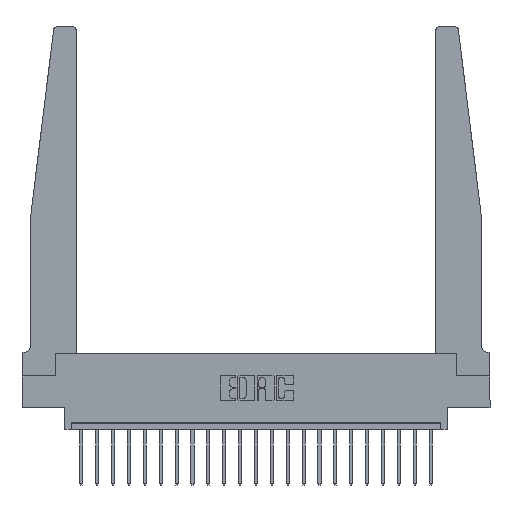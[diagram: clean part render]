
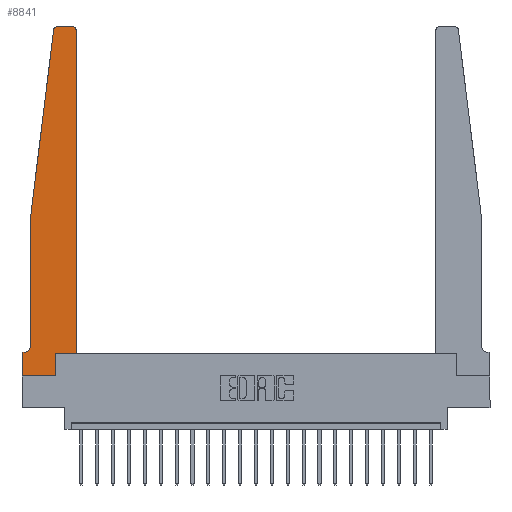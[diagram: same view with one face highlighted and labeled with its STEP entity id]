
A CAD part, top view. The second image highlights one B-rep face of the part: STEP entity #8841.
In plain terms, the highlighted planar face has unit normal (0, 0, 1).
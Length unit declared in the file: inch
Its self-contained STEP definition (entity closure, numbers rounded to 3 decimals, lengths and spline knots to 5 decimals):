
#238 = VECTOR ( 'NONE', #19672, 39.37008 ) ;
#254 = CARTESIAN_POINT ( 'NONE',  ( 0.065, 0.1875, 0.37 ) ) ;
#684 = CARTESIAN_POINT ( 'NONE',  ( 0.425, 0.18, 0.37 ) ) ;
#1809 = LINE ( 'NONE', #3387, #8840 ) ;
#2019 = LINE ( 'NONE', #8628, #5111 ) ;
#2046 = DIRECTION ( 'NONE',  ( 0., 1., 0. ) ) ;
#2198 = EDGE_CURVE ( 'NONE', #18821, #7153, #13182, .T. ) ;
#2210 = CARTESIAN_POINT ( 'NONE',  ( 0., 0.1875, 0.37 ) ) ;
#2639 = CARTESIAN_POINT ( 'NONE',  ( 0.065, 1.25, 0.37 ) ) ;
#3086 = CARTESIAN_POINT ( 'NONE',  ( 0., 0., 0.37 ) ) ;
#3207 = EDGE_CURVE ( 'NONE', #20640, #17232, #13992, .T. ) ;
#3245 = EDGE_CURVE ( 'NONE', #11460, #18821, #2019, .T. ) ;
#3387 = CARTESIAN_POINT ( 'NONE',  ( 0., 0., 0.37 ) ) ;
#3654 = CARTESIAN_POINT ( 'NONE',  ( 0.425, 0.18, 0.37 ) ) ;
#3696 = ORIENTED_EDGE ( 'NONE', *, *, #17014, .T. ) ;
#4176 = VERTEX_POINT ( 'NONE', #3654 ) ;
#4183 = ORIENTED_EDGE ( 'NONE', *, *, #4213, .T. ) ;
#4193 = CARTESIAN_POINT ( 'NONE',  ( 0., 0., 0.37 ) ) ;
#4213 = EDGE_CURVE ( 'NONE', #21275, #11460, #18660, .T. ) ;
#4415 = VECTOR ( 'NONE', #19934, 39.37008 ) ;
#4631 = DIRECTION ( 'NONE',  ( 0., 0., 1. ) ) ;
#4739 = CARTESIAN_POINT ( 'NONE',  ( 0.2605, 0.18, 0.37 ) ) ;
#5111 = VECTOR ( 'NONE', #20880, 39.37008 ) ;
#5242 = CIRCLE ( 'NONE', #5597, 0.05 ) ;
#5386 = ORIENTED_EDGE ( 'NONE', *, *, #16662, .T. ) ;
#5497 = ORIENTED_EDGE ( 'NONE', *, *, #6106, .T. ) ;
#5597 = AXIS2_PLACEMENT_3D ( 'NONE', #15223, #18388, #20542 ) ;
#5650 = VERTEX_POINT ( 'NONE', #10037 ) ;
#5939 = ORIENTED_EDGE ( 'NONE', *, *, #6409, .T. ) ;
#6106 = EDGE_CURVE ( 'NONE', #6944, #18657, #12015, .T. ) ;
#6140 = ORIENTED_EDGE ( 'NONE', *, *, #19120, .T. ) ;
#6233 = LINE ( 'NONE', #13050, #4415 ) ;
#6409 = EDGE_CURVE ( 'NONE', #13388, #5650, #11427, .T. ) ;
#6418 = DIRECTION ( 'NONE',  ( 0., -1., 0. ) ) ;
#6906 = CARTESIAN_POINT ( 'NONE',  ( 0.015, 0.1875, 0.37 ) ) ;
#6944 = VERTEX_POINT ( 'NONE', #6906 ) ;
#7153 = VERTEX_POINT ( 'NONE', #18209 ) ;
#8007 = DIRECTION ( 'NONE',  ( 0., 0., 1. ) ) ;
#8098 = FACE_OUTER_BOUND ( 'NONE', #16474, .T. ) ;
#8628 = CARTESIAN_POINT ( 'NONE',  ( 0.065, 1.25, 0.37 ) ) ;
#8840 = VECTOR ( 'NONE', #6418, 39.37008 ) ;
#8841 = ADVANCED_FACE ( 'NONE', ( #8098 ), #9337, .T. ) ;
#8883 = DIRECTION ( 'NONE',  ( -1., 0., 0. ) ) ;
#9337 = PLANE ( 'NONE',  #18288 ) ;
#9798 = CARTESIAN_POINT ( 'NONE',  ( 0.24675, 2.72367, 0.37 ) ) ;
#9815 = VERTEX_POINT ( 'NONE', #3086 ) ;
#10037 = CARTESIAN_POINT ( 'NONE',  ( 0.2605, 0.18, 0.37 ) ) ;
#10525 = DIRECTION ( 'NONE',  ( 0., 0., 1. ) ) ;
#10931 = VECTOR ( 'NONE', #15127, 39.37008 ) ;
#11115 = DIRECTION ( 'NONE',  ( 1., 0., 0. ) ) ;
#11427 = LINE ( 'NONE', #4739, #10931 ) ;
#11460 = VERTEX_POINT ( 'NONE', #9798 ) ;
#11615 = DIRECTION ( 'NONE',  ( 0., -1., 0. ) ) ;
#11691 = VECTOR ( 'NONE', #8883, 39.37008 ) ;
#11866 = CARTESIAN_POINT ( 'NONE',  ( 0.395, 2.72, 0.37 ) ) ;
#12015 = LINE ( 'NONE', #254, #11691 ) ;
#12471 = LINE ( 'NONE', #19565, #13439 ) ;
#12671 = CARTESIAN_POINT ( 'NONE',  ( 0., 0.1875, 0.37 ) ) ;
#12743 = EDGE_CURVE ( 'NONE', #17232, #21275, #6233, .T. ) ;
#13050 = CARTESIAN_POINT ( 'NONE',  ( 0.25, 2.75, 0.37 ) ) ;
#13182 = LINE ( 'NONE', #20069, #17955 ) ;
#13388 = VERTEX_POINT ( 'NONE', #17697 ) ;
#13439 = VECTOR ( 'NONE', #11115, 39.37008 ) ;
#13992 = CIRCLE ( 'NONE', #20852, 0.03 ) ;
#14015 = LINE ( 'NONE', #684, #18488 ) ;
#14582 = ORIENTED_EDGE ( 'NONE', *, *, #17688, .T. ) ;
#15127 = DIRECTION ( 'NONE',  ( 0., 1., 0. ) ) ;
#15223 = CARTESIAN_POINT ( 'NONE',  ( 0.015, 0.2375, 0.37 ) ) ;
#15517 = ORIENTED_EDGE ( 'NONE', *, *, #3207, .T. ) ;
#16293 = ORIENTED_EDGE ( 'NONE', *, *, #17976, .T. ) ;
#16474 = EDGE_LOOP ( 'NONE', ( #18434, #4183, #20527, #17191, #16293, #5497, #14582, #6140, #5939, #5386, #3696, #15517 ) ) ;
#16515 = CARTESIAN_POINT ( 'NONE',  ( 0.27653, 2.72, 0.37 ) ) ;
#16662 = EDGE_CURVE ( 'NONE', #5650, #4176, #12471, .T. ) ;
#16954 = CARTESIAN_POINT ( 'NONE',  ( 0.425, 2.72, 0.37 ) ) ;
#17014 = EDGE_CURVE ( 'NONE', #4176, #20640, #14015, .T. ) ;
#17191 = ORIENTED_EDGE ( 'NONE', *, *, #2198, .T. ) ;
#17232 = VERTEX_POINT ( 'NONE', #19056 ) ;
#17688 = EDGE_CURVE ( 'NONE', #18657, #9815, #1809, .T. ) ;
#17697 = CARTESIAN_POINT ( 'NONE',  ( 0.2605, 0., 0.37 ) ) ;
#17935 = CARTESIAN_POINT ( 'NONE',  ( 0.27653, 2.75, 0.37 ) ) ;
#17955 = VECTOR ( 'NONE', #11615, 39.37008 ) ;
#17973 = LINE ( 'NONE', #4193, #238 ) ;
#17976 = EDGE_CURVE ( 'NONE', #7153, #6944, #5242, .T. ) ;
#18209 = CARTESIAN_POINT ( 'NONE',  ( 0.065, 0.2375, 0.37 ) ) ;
#18288 = AXIS2_PLACEMENT_3D ( 'NONE', #12671, #4631, #19547 ) ;
#18388 = DIRECTION ( 'NONE',  ( 0., 0., -1. ) ) ;
#18434 = ORIENTED_EDGE ( 'NONE', *, *, #12743, .T. ) ;
#18488 = VECTOR ( 'NONE', #2046, 39.37008 ) ;
#18657 = VERTEX_POINT ( 'NONE', #2210 ) ;
#18660 = CIRCLE ( 'NONE', #20121, 0.03 ) ;
#18726 = DIRECTION ( 'NONE',  ( 1., 0., 0. ) ) ;
#18821 = VERTEX_POINT ( 'NONE', #2639 ) ;
#19056 = CARTESIAN_POINT ( 'NONE',  ( 0.395, 2.75, 0.37 ) ) ;
#19120 = EDGE_CURVE ( 'NONE', #9815, #13388, #17973, .T. ) ;
#19547 = DIRECTION ( 'NONE',  ( 1., 0., 0. ) ) ;
#19565 = CARTESIAN_POINT ( 'NONE',  ( 0.425, 0.18, 0.37 ) ) ;
#19672 = DIRECTION ( 'NONE',  ( 1., 0., 0. ) ) ;
#19934 = DIRECTION ( 'NONE',  ( -1., 0., 0. ) ) ;
#20019 = DIRECTION ( 'NONE',  ( 1., 0., 0. ) ) ;
#20069 = CARTESIAN_POINT ( 'NONE',  ( 0.065, 1.25, 0.37 ) ) ;
#20121 = AXIS2_PLACEMENT_3D ( 'NONE', #16515, #8007, #20019 ) ;
#20527 = ORIENTED_EDGE ( 'NONE', *, *, #3245, .T. ) ;
#20542 = DIRECTION ( 'NONE',  ( -1., 0., 0. ) ) ;
#20640 = VERTEX_POINT ( 'NONE', #16954 ) ;
#20852 = AXIS2_PLACEMENT_3D ( 'NONE', #11866, #10525, #18726 ) ;
#20880 = DIRECTION ( 'NONE',  ( -0.122, -0.992, 0. ) ) ;
#21275 = VERTEX_POINT ( 'NONE', #17935 ) ;
